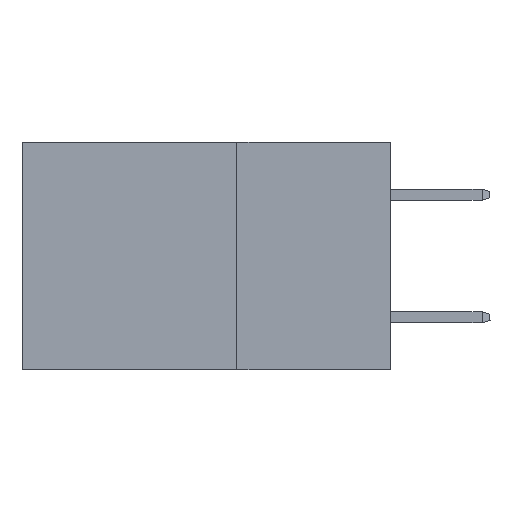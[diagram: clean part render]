
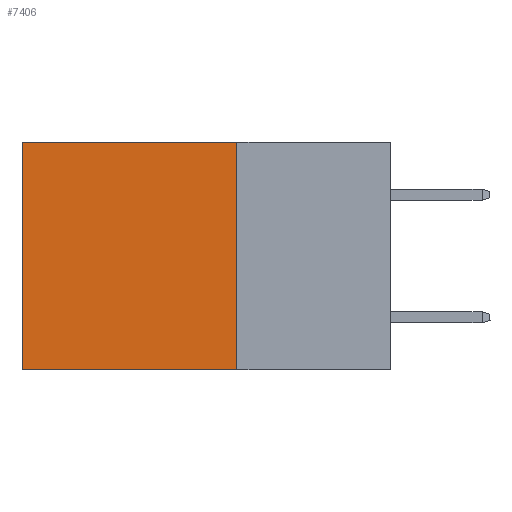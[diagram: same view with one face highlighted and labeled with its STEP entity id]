
A CAD part, left-side view. The second image highlights one B-rep face of the part: STEP entity #7406.
In plain terms, the highlighted planar face has unit normal (-1, 0, 0).
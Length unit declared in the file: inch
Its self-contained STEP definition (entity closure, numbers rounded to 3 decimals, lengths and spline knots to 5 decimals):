
#654 = EDGE_CURVE ( 'NONE', #17283, #14932, #18229, .T. ) ;
#783 = DIRECTION ( 'NONE',  ( 0., 0., -1. ) ) ;
#1742 = ORIENTED_EDGE ( 'NONE', *, *, #9983, .F. ) ;
#1882 = DIRECTION ( 'NONE',  ( 0., 1., 0. ) ) ;
#2630 = CARTESIAN_POINT ( 'NONE',  ( 0.2875, 0.25, 0. ) ) ;
#2921 = LINE ( 'NONE', #14982, #21496 ) ;
#3113 = CARTESIAN_POINT ( 'NONE',  ( 0.2875, 0.6, 0. ) ) ;
#3291 = EDGE_CURVE ( 'NONE', #5748, #19695, #2921, .T. ) ;
#4081 = FACE_OUTER_BOUND ( 'NONE', #19236, .T. ) ;
#4272 = LINE ( 'NONE', #9114, #22302 ) ;
#4327 = ORIENTED_EDGE ( 'NONE', *, *, #654, .F. ) ;
#4738 = CARTESIAN_POINT ( 'NONE',  ( 0.2875, 0.25, 0. ) ) ;
#4856 = ORIENTED_EDGE ( 'NONE', *, *, #3291, .T. ) ;
#4920 = EDGE_CURVE ( 'NONE', #17283, #5748, #12903, .T. ) ;
#5748 = VERTEX_POINT ( 'NONE', #3113 ) ;
#6773 = CARTESIAN_POINT ( 'NONE',  ( 0.2875, 0.25, 0. ) ) ;
#7406 = ADVANCED_FACE ( 'NONE', ( #4081 ), #17243, .F. ) ;
#8489 = AXIS2_PLACEMENT_3D ( 'NONE', #6773, #21206, #17874 ) ;
#9114 = CARTESIAN_POINT ( 'NONE',  ( 0.2875, 0.25, -0.37 ) ) ;
#9983 = EDGE_CURVE ( 'NONE', #14932, #19695, #4272, .T. ) ;
#11590 = ORIENTED_EDGE ( 'NONE', *, *, #4920, .T. ) ;
#12903 = LINE ( 'NONE', #21007, #13477 ) ;
#13477 = VECTOR ( 'NONE', #13940, 39.37008 ) ;
#13940 = DIRECTION ( 'NONE',  ( 0., 1., 0. ) ) ;
#14932 = VERTEX_POINT ( 'NONE', #17597 ) ;
#14982 = CARTESIAN_POINT ( 'NONE',  ( 0.2875, 0.6, 0. ) ) ;
#15660 = DIRECTION ( 'NONE',  ( 0., 0., -1. ) ) ;
#17243 = PLANE ( 'NONE',  #8489 ) ;
#17283 = VERTEX_POINT ( 'NONE', #2630 ) ;
#17581 = CARTESIAN_POINT ( 'NONE',  ( 0.2875, 0.6, -0.37 ) ) ;
#17597 = CARTESIAN_POINT ( 'NONE',  ( 0.2875, 0.25, -0.37 ) ) ;
#17651 = VECTOR ( 'NONE', #15660, 39.37008 ) ;
#17874 = DIRECTION ( 'NONE',  ( 0., 0., -1. ) ) ;
#18229 = LINE ( 'NONE', #4738, #17651 ) ;
#19236 = EDGE_LOOP ( 'NONE', ( #4856, #1742, #4327, #11590 ) ) ;
#19695 = VERTEX_POINT ( 'NONE', #17581 ) ;
#21007 = CARTESIAN_POINT ( 'NONE',  ( 0.2875, 0.25, 0. ) ) ;
#21206 = DIRECTION ( 'NONE',  ( 1., 0., 0. ) ) ;
#21496 = VECTOR ( 'NONE', #783, 39.37008 ) ;
#22302 = VECTOR ( 'NONE', #1882, 39.37008 ) ;
